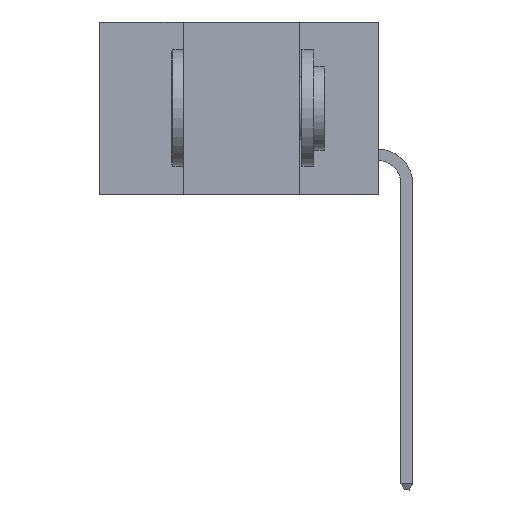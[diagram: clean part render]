
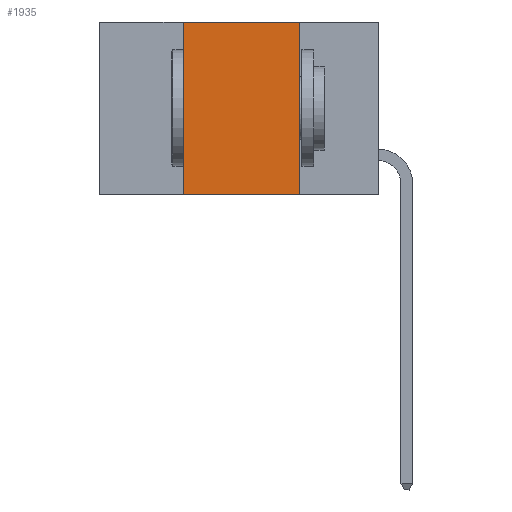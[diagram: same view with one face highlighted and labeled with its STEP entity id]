
A CAD part, left-side view. The second image highlights one B-rep face of the part: STEP entity #1935.
In plain terms, the highlighted planar face has unit normal (-1, 0, 0).
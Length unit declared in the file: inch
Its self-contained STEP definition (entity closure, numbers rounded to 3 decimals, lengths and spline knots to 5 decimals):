
#399 = CARTESIAN_POINT ( 'NONE',  ( 0., 0.17, -0.37 ) ) ;
#798 = ORIENTED_EDGE ( 'NONE', *, *, #10321, .F. ) ;
#968 = VERTEX_POINT ( 'NONE', #9079 ) ;
#1935 = ADVANCED_FACE ( 'NONE', ( #3491 ), #16587, .F. ) ;
#2366 = VECTOR ( 'NONE', #15208, 39.37008 ) ;
#3491 = FACE_OUTER_BOUND ( 'NONE', #6353, .T. ) ;
#4378 = DIRECTION ( 'NONE',  ( 0., 0., -1. ) ) ;
#4451 = CARTESIAN_POINT ( 'NONE',  ( 0., 0.6, -0.37 ) ) ;
#4545 = DIRECTION ( 'NONE',  ( 0., 0., -1. ) ) ;
#4680 = LINE ( 'NONE', #4451, #2366 ) ;
#4753 = AXIS2_PLACEMENT_3D ( 'NONE', #8564, #11253, #4545 ) ;
#5113 = CARTESIAN_POINT ( 'NONE',  ( 0., 0.42, 0. ) ) ;
#5472 = LINE ( 'NONE', #6946, #15290 ) ;
#5570 = LINE ( 'NONE', #13237, #12070 ) ;
#6353 = EDGE_LOOP ( 'NONE', ( #11063, #8613, #798, #7371 ) ) ;
#6946 = CARTESIAN_POINT ( 'NONE',  ( 0., 0.17, 0. ) ) ;
#7371 = ORIENTED_EDGE ( 'NONE', *, *, #9078, .T. ) ;
#7625 = LINE ( 'NONE', #5113, #16999 ) ;
#7850 = VERTEX_POINT ( 'NONE', #17260 ) ;
#8141 = EDGE_CURVE ( 'NONE', #8887, #7850, #5570, .T. ) ;
#8544 = CARTESIAN_POINT ( 'NONE',  ( 0., 0.42, 0. ) ) ;
#8564 = CARTESIAN_POINT ( 'NONE',  ( 0., 0.6, 0. ) ) ;
#8613 = ORIENTED_EDGE ( 'NONE', *, *, #8141, .F. ) ;
#8887 = VERTEX_POINT ( 'NONE', #8544 ) ;
#9078 = EDGE_CURVE ( 'NONE', #968, #11963, #4680, .T. ) ;
#9079 = CARTESIAN_POINT ( 'NONE',  ( 0., 0.42, -0.37 ) ) ;
#10321 = EDGE_CURVE ( 'NONE', #968, #8887, #7625, .T. ) ;
#11063 = ORIENTED_EDGE ( 'NONE', *, *, #11299, .F. ) ;
#11253 = DIRECTION ( 'NONE',  ( 1., 0., 0. ) ) ;
#11299 = EDGE_CURVE ( 'NONE', #7850, #11963, #5472, .T. ) ;
#11963 = VERTEX_POINT ( 'NONE', #399 ) ;
#12070 = VECTOR ( 'NONE', #16357, 39.37008 ) ;
#13237 = CARTESIAN_POINT ( 'NONE',  ( 0., 0.6, 0. ) ) ;
#15208 = DIRECTION ( 'NONE',  ( 0., -1., 0. ) ) ;
#15290 = VECTOR ( 'NONE', #4378, 39.37008 ) ;
#15387 = DIRECTION ( 'NONE',  ( 0., 0., 1. ) ) ;
#16357 = DIRECTION ( 'NONE',  ( 0., -1., 0. ) ) ;
#16587 = PLANE ( 'NONE',  #4753 ) ;
#16999 = VECTOR ( 'NONE', #15387, 39.37008 ) ;
#17260 = CARTESIAN_POINT ( 'NONE',  ( 0., 0.17, 0. ) ) ;
